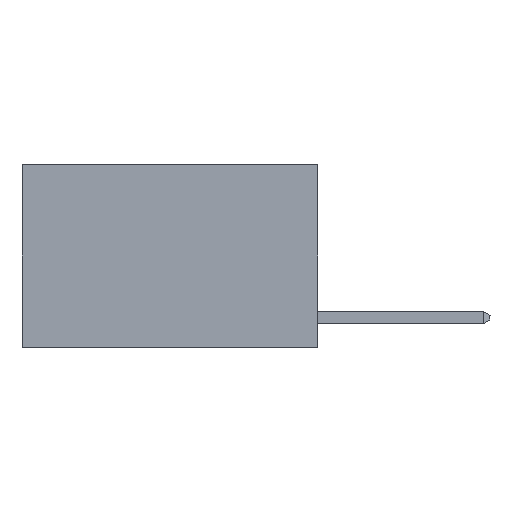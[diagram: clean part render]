
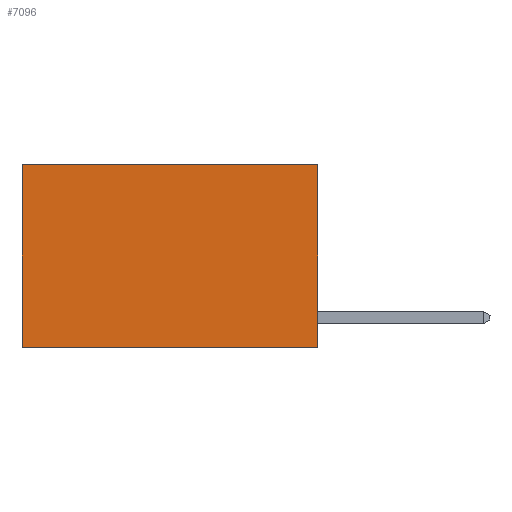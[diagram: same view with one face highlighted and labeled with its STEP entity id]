
A CAD part, left-side view. The second image highlights one B-rep face of the part: STEP entity #7096.
In plain terms, the highlighted planar face has unit normal (-1, 0, 0).
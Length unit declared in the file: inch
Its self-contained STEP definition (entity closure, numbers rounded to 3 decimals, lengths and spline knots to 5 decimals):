
#167 = EDGE_CURVE ( 'NONE', #10938, #2806, #7419, .T. ) ;
#219 = EDGE_CURVE ( 'NONE', #10938, #6071, #9159, .T. ) ;
#348 = VECTOR ( 'NONE', #3131, 39.37008 ) ;
#372 = DIRECTION ( 'NONE',  ( 0., 0., -1. ) ) ;
#819 = VERTEX_POINT ( 'NONE', #5268 ) ;
#1510 = ORIENTED_EDGE ( 'NONE', *, *, #167, .F. ) ;
#1534 = DIRECTION ( 'NONE',  ( 1., 0., 0. ) ) ;
#1578 = CARTESIAN_POINT ( 'NONE',  ( 0.2625, 0., -0.37 ) ) ;
#2455 = ORIENTED_EDGE ( 'NONE', *, *, #219, .T. ) ;
#2806 = VERTEX_POINT ( 'NONE', #3336 ) ;
#2857 = CARTESIAN_POINT ( 'NONE',  ( 0.2625, 0., 0. ) ) ;
#3131 = DIRECTION ( 'NONE',  ( 0., 0., -1. ) ) ;
#3336 = CARTESIAN_POINT ( 'NONE',  ( 0.2625, 0., -0.37 ) ) ;
#3949 = DIRECTION ( 'NONE',  ( 0., 1., 0. ) ) ;
#4360 = VECTOR ( 'NONE', #3949, 39.37008 ) ;
#4663 = CARTESIAN_POINT ( 'NONE',  ( 0.2625, 0.6, 0. ) ) ;
#5156 = ORIENTED_EDGE ( 'NONE', *, *, #6403, .F. ) ;
#5268 = CARTESIAN_POINT ( 'NONE',  ( 0.2625, 0.6, -0.37 ) ) ;
#5799 = CARTESIAN_POINT ( 'NONE',  ( 0.2625, 0., 0. ) ) ;
#5859 = PLANE ( 'NONE',  #7601 ) ;
#5889 = VECTOR ( 'NONE', #10288, 39.37008 ) ;
#6071 = VERTEX_POINT ( 'NONE', #8645 ) ;
#6403 = EDGE_CURVE ( 'NONE', #2806, #819, #8342, .T. ) ;
#7025 = FACE_OUTER_BOUND ( 'NONE', #9409, .T. ) ;
#7096 = ADVANCED_FACE ( 'NONE', ( #7025 ), #5859, .F. ) ;
#7419 = LINE ( 'NONE', #2857, #348 ) ;
#7601 = AXIS2_PLACEMENT_3D ( 'NONE', #9377, #1534, #7761 ) ;
#7761 = DIRECTION ( 'NONE',  ( 0., 0., -1. ) ) ;
#8342 = LINE ( 'NONE', #1578, #5889 ) ;
#8497 = VECTOR ( 'NONE', #372, 39.37008 ) ;
#8645 = CARTESIAN_POINT ( 'NONE',  ( 0.2625, 0.6, 0. ) ) ;
#9159 = LINE ( 'NONE', #5799, #4360 ) ;
#9377 = CARTESIAN_POINT ( 'NONE',  ( 0.2625, 0., 0. ) ) ;
#9409 = EDGE_LOOP ( 'NONE', ( #11102, #5156, #1510, #2455 ) ) ;
#10288 = DIRECTION ( 'NONE',  ( 0., 1., 0. ) ) ;
#10697 = CARTESIAN_POINT ( 'NONE',  ( 0.2625, 0., 0. ) ) ;
#10911 = LINE ( 'NONE', #4663, #8497 ) ;
#10938 = VERTEX_POINT ( 'NONE', #10697 ) ;
#11021 = EDGE_CURVE ( 'NONE', #6071, #819, #10911, .T. ) ;
#11102 = ORIENTED_EDGE ( 'NONE', *, *, #11021, .T. ) ;
